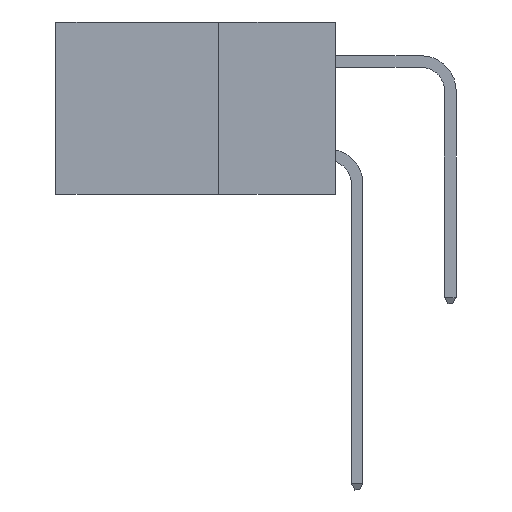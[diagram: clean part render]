
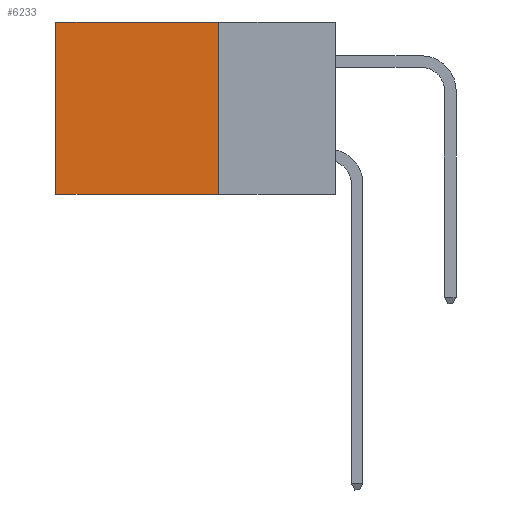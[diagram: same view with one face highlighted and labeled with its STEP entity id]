
A CAD part, left-side view. The second image highlights one B-rep face of the part: STEP entity #6233.
In plain terms, the highlighted planar face has unit normal (-1, 0, 0).
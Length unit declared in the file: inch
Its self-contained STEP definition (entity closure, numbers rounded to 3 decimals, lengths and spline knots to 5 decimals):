
#647 = EDGE_CURVE ( 'NONE', #17953, #21393, #17317, .T. ) ;
#1577 = FACE_OUTER_BOUND ( 'NONE', #21031, .T. ) ;
#1828 = LINE ( 'NONE', #13456, #21182 ) ;
#3289 = VERTEX_POINT ( 'NONE', #14272 ) ;
#4323 = ORIENTED_EDGE ( 'NONE', *, *, #647, .F. ) ;
#4387 = CARTESIAN_POINT ( 'NONE',  ( 0.2875, 0.25, 0. ) ) ;
#4512 = DIRECTION ( 'NONE',  ( 0., 1., 0. ) ) ;
#4732 = VECTOR ( 'NONE', #4512, 39.37008 ) ;
#4819 = ORIENTED_EDGE ( 'NONE', *, *, #19769, .T. ) ;
#6233 = ADVANCED_FACE ( 'NONE', ( #1577 ), #16895, .F. ) ;
#7044 = EDGE_CURVE ( 'NONE', #3289, #21393, #22579, .T. ) ;
#9880 = CARTESIAN_POINT ( 'NONE',  ( 0.2875, 0.25, -0.37 ) ) ;
#9923 = CARTESIAN_POINT ( 'NONE',  ( 0.2875, 0.6, 0. ) ) ;
#10236 = LINE ( 'NONE', #4387, #14642 ) ;
#10654 = VERTEX_POINT ( 'NONE', #21871 ) ;
#13237 = DIRECTION ( 'NONE',  ( 0., 0., -1. ) ) ;
#13456 = CARTESIAN_POINT ( 'NONE',  ( 0.2875, 0.25, 0. ) ) ;
#14025 = CARTESIAN_POINT ( 'NONE',  ( 0.2875, 0.25, -0.37 ) ) ;
#14241 = CARTESIAN_POINT ( 'NONE',  ( 0.2875, 0.6, -0.37 ) ) ;
#14272 = CARTESIAN_POINT ( 'NONE',  ( 0.2875, 0.6, 0. ) ) ;
#14642 = VECTOR ( 'NONE', #15624, 39.37008 ) ;
#15493 = DIRECTION ( 'NONE',  ( 0., 0., -1. ) ) ;
#15624 = DIRECTION ( 'NONE',  ( 0., 0., -1. ) ) ;
#16895 = PLANE ( 'NONE',  #17644 ) ;
#17317 = LINE ( 'NONE', #9880, #4732 ) ;
#17644 = AXIS2_PLACEMENT_3D ( 'NONE', #22383, #24124, #13237 ) ;
#17780 = VECTOR ( 'NONE', #15493, 39.37008 ) ;
#17953 = VERTEX_POINT ( 'NONE', #14025 ) ;
#18556 = EDGE_CURVE ( 'NONE', #10654, #17953, #10236, .T. ) ;
#19769 = EDGE_CURVE ( 'NONE', #10654, #3289, #1828, .T. ) ;
#20684 = ORIENTED_EDGE ( 'NONE', *, *, #18556, .F. ) ;
#20869 = DIRECTION ( 'NONE',  ( 0., 1., 0. ) ) ;
#21031 = EDGE_LOOP ( 'NONE', ( #21818, #4323, #20684, #4819 ) ) ;
#21182 = VECTOR ( 'NONE', #20869, 39.37008 ) ;
#21393 = VERTEX_POINT ( 'NONE', #14241 ) ;
#21818 = ORIENTED_EDGE ( 'NONE', *, *, #7044, .T. ) ;
#21871 = CARTESIAN_POINT ( 'NONE',  ( 0.2875, 0.25, 0. ) ) ;
#22383 = CARTESIAN_POINT ( 'NONE',  ( 0.2875, 0.25, 0. ) ) ;
#22579 = LINE ( 'NONE', #9923, #17780 ) ;
#24124 = DIRECTION ( 'NONE',  ( 1., 0., 0. ) ) ;
